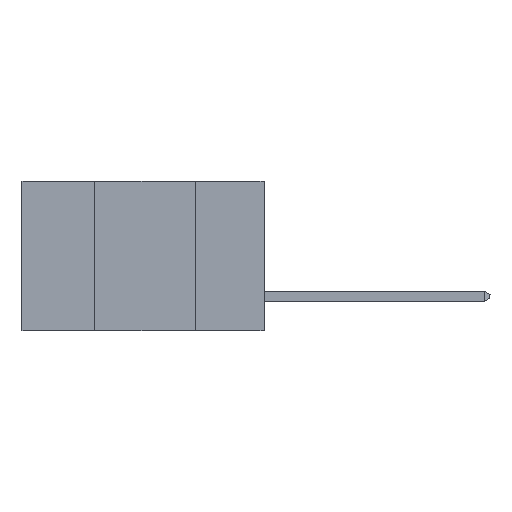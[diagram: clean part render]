
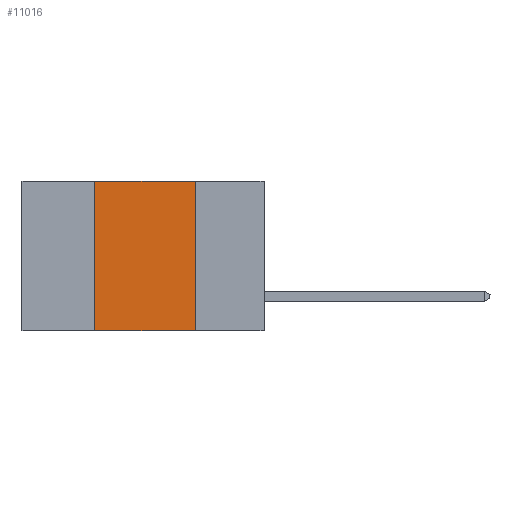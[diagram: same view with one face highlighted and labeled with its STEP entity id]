
A CAD part, left-side view. The second image highlights one B-rep face of the part: STEP entity #11016.
In plain terms, the highlighted planar face has unit normal (-1, 0, 0).
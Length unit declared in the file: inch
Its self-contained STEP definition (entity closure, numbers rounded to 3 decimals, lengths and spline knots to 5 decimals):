
#457 = CARTESIAN_POINT ( 'NONE',  ( 0., 0.6, 0. ) ) ;
#848 = EDGE_LOOP ( 'NONE', ( #4181, #25259, #19846, #25339 ) ) ;
#2400 = VERTEX_POINT ( 'NONE', #12461 ) ;
#3521 = FACE_OUTER_BOUND ( 'NONE', #848, .T. ) ;
#3765 = LINE ( 'NONE', #4556, #23115 ) ;
#4181 = ORIENTED_EDGE ( 'NONE', *, *, #25736, .F. ) ;
#4556 = CARTESIAN_POINT ( 'NONE',  ( 0., 0.6, -0.37 ) ) ;
#4580 = EDGE_CURVE ( 'NONE', #7949, #10219, #11988, .T. ) ;
#5677 = CARTESIAN_POINT ( 'NONE',  ( 0., 0.17, -0.37 ) ) ;
#5737 = EDGE_CURVE ( 'NONE', #2400, #7949, #13487, .T. ) ;
#7949 = VERTEX_POINT ( 'NONE', #15059 ) ;
#8332 = DIRECTION ( 'NONE',  ( 1., 0., 0. ) ) ;
#8416 = PLANE ( 'NONE',  #12409 ) ;
#9345 = DIRECTION ( 'NONE',  ( 0., -1., 0. ) ) ;
#10219 = VERTEX_POINT ( 'NONE', #25788 ) ;
#10991 = DIRECTION ( 'NONE',  ( 0., 0., 1. ) ) ;
#11016 = ADVANCED_FACE ( 'NONE', ( #3521 ), #8416, .F. ) ;
#11307 = DIRECTION ( 'NONE',  ( 0., 0., -1. ) ) ;
#11988 = LINE ( 'NONE', #21825, #16951 ) ;
#12409 = AXIS2_PLACEMENT_3D ( 'NONE', #457, #8332, #14402 ) ;
#12461 = CARTESIAN_POINT ( 'NONE',  ( 0., 0.42, -0.37 ) ) ;
#13487 = LINE ( 'NONE', #14798, #24432 ) ;
#14402 = DIRECTION ( 'NONE',  ( 0., 0., -1. ) ) ;
#14798 = CARTESIAN_POINT ( 'NONE',  ( 0., 0.42, 0. ) ) ;
#15059 = CARTESIAN_POINT ( 'NONE',  ( 0., 0.42, 0. ) ) ;
#16256 = EDGE_CURVE ( 'NONE', #2400, #16911, #3765, .T. ) ;
#16702 = VECTOR ( 'NONE', #11307, 39.37008 ) ;
#16911 = VERTEX_POINT ( 'NONE', #5677 ) ;
#16951 = VECTOR ( 'NONE', #17869, 39.37008 ) ;
#17869 = DIRECTION ( 'NONE',  ( 0., -1., 0. ) ) ;
#19491 = LINE ( 'NONE', #20966, #16702 ) ;
#19846 = ORIENTED_EDGE ( 'NONE', *, *, #5737, .F. ) ;
#20966 = CARTESIAN_POINT ( 'NONE',  ( 0., 0.17, 0. ) ) ;
#21825 = CARTESIAN_POINT ( 'NONE',  ( 0., 0.6, 0. ) ) ;
#23115 = VECTOR ( 'NONE', #9345, 39.37008 ) ;
#24432 = VECTOR ( 'NONE', #10991, 39.37008 ) ;
#25259 = ORIENTED_EDGE ( 'NONE', *, *, #4580, .F. ) ;
#25339 = ORIENTED_EDGE ( 'NONE', *, *, #16256, .T. ) ;
#25736 = EDGE_CURVE ( 'NONE', #10219, #16911, #19491, .T. ) ;
#25788 = CARTESIAN_POINT ( 'NONE',  ( 0., 0.17, 0. ) ) ;
